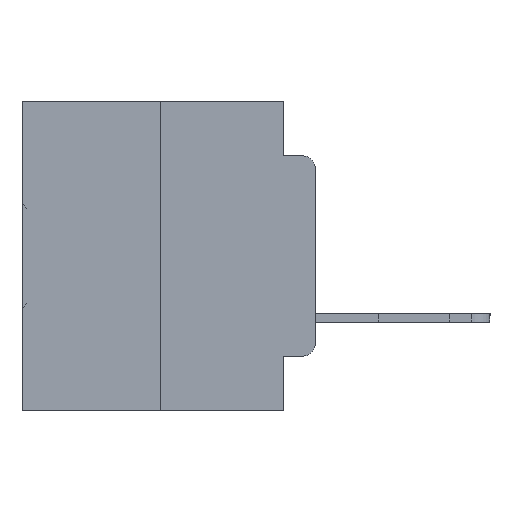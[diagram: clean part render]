
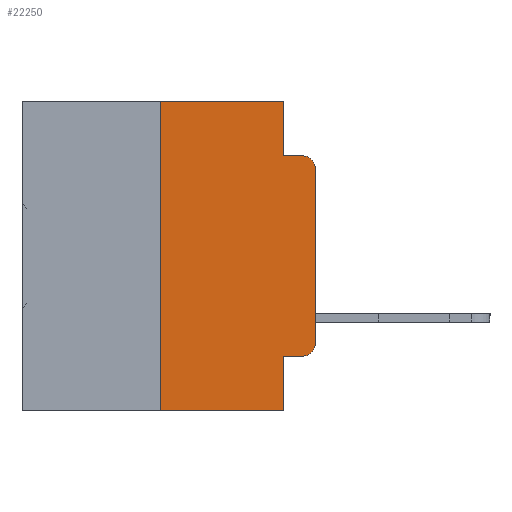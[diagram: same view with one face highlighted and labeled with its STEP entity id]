
A CAD part, left-side view. The second image highlights one B-rep face of the part: STEP entity #22250.
In plain terms, the highlighted planar face has unit normal (-1, 0, 0).
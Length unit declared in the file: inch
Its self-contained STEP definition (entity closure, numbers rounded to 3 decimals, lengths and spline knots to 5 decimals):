
#383 = CARTESIAN_POINT ( 'NONE',  ( 0., 0., -0.1085 ) ) ;
#525 = PLANE ( 'NONE',  #16255 ) ;
#553 = CARTESIAN_POINT ( 'NONE',  ( 0., 0.02, -0.3915 ) ) ;
#1141 = EDGE_CURVE ( 'NONE', #23824, #31234, #19177, .T. ) ;
#1585 = DIRECTION ( 'NONE',  ( 0., -1., 0. ) ) ;
#1615 = FACE_OUTER_BOUND ( 'NONE', #7427, .T. ) ;
#2001 = VECTOR ( 'NONE', #4054, 39.37008 ) ;
#2354 = ORIENTED_EDGE ( 'NONE', *, *, #4881, .T. ) ;
#2750 = VERTEX_POINT ( 'NONE', #25163 ) ;
#2858 = LINE ( 'NONE', #28061, #2001 ) ;
#3004 = EDGE_CURVE ( 'NONE', #31234, #20002, #31728, .T. ) ;
#3351 = DIRECTION ( 'NONE',  ( 0., 0., -1. ) ) ;
#3569 = DIRECTION ( 'NONE',  ( 0., 0., -1. ) ) ;
#4054 = DIRECTION ( 'NONE',  ( 0., 0., 1. ) ) ;
#4753 = VECTOR ( 'NONE', #26905, 39.37008 ) ;
#4881 = EDGE_CURVE ( 'NONE', #18666, #20002, #23552, .T. ) ;
#5510 = DIRECTION ( 'NONE',  ( -1., 0., 0. ) ) ;
#5546 = CARTESIAN_POINT ( 'NONE',  ( 0., 0.051, 0. ) ) ;
#5762 = CARTESIAN_POINT ( 'NONE',  ( 0., 0., 0. ) ) ;
#6622 = VECTOR ( 'NONE', #24027, 39.37008 ) ;
#6734 = EDGE_CURVE ( 'NONE', #2750, #18666, #7289, .T. ) ;
#7289 = LINE ( 'NONE', #5762, #8996 ) ;
#7427 = EDGE_LOOP ( 'NONE', ( #26678, #2354, #27138, #8411, #12592, #12186, #31841, #19689, #21334, #31044 ) ) ;
#8411 = ORIENTED_EDGE ( 'NONE', *, *, #1141, .F. ) ;
#8996 = VECTOR ( 'NONE', #24413, 39.37008 ) ;
#9454 = LINE ( 'NONE', #23056, #22681 ) ;
#9688 = VECTOR ( 'NONE', #33316, 39.37008 ) ;
#10018 = CIRCLE ( 'NONE', #17502, 0.02 ) ;
#11659 = CARTESIAN_POINT ( 'NONE',  ( 0., 0.473, 0. ) ) ;
#12150 = VECTOR ( 'NONE', #23650, 39.37008 ) ;
#12186 = ORIENTED_EDGE ( 'NONE', *, *, #30680, .F. ) ;
#12581 = EDGE_CURVE ( 'NONE', #21993, #22025, #9454, .T. ) ;
#12592 = ORIENTED_EDGE ( 'NONE', *, *, #18790, .F. ) ;
#13046 = CARTESIAN_POINT ( 'NONE',  ( 0., 0.051, 0. ) ) ;
#13049 = CARTESIAN_POINT ( 'NONE',  ( 0., 0.051, 0. ) ) ;
#14512 = CARTESIAN_POINT ( 'NONE',  ( 0., 0.473, 0. ) ) ;
#15523 = DIRECTION ( 'NONE',  ( 0., -1., 0. ) ) ;
#16255 = AXIS2_PLACEMENT_3D ( 'NONE', #11659, #19620, #3569 ) ;
#16707 = LINE ( 'NONE', #14512, #9688 ) ;
#16954 = AXIS2_PLACEMENT_3D ( 'NONE', #21490, #5510, #24166 ) ;
#17208 = CARTESIAN_POINT ( 'NONE',  ( 0., 0.02, -0.0885 ) ) ;
#17502 = AXIS2_PLACEMENT_3D ( 'NONE', #553, #19426, #3351 ) ;
#18666 = VERTEX_POINT ( 'NONE', #383 ) ;
#18790 = EDGE_CURVE ( 'NONE', #25694, #23824, #16707, .T. ) ;
#19177 = LINE ( 'NONE', #13046, #12150 ) ;
#19426 = DIRECTION ( 'NONE',  ( -1., 0., 0. ) ) ;
#19620 = DIRECTION ( 'NONE',  ( 1., 0., 0. ) ) ;
#19689 = ORIENTED_EDGE ( 'NONE', *, *, #28872, .F. ) ;
#19875 = EDGE_CURVE ( 'NONE', #29546, #2750, #10018, .T. ) ;
#19976 = CARTESIAN_POINT ( 'NONE',  ( 0., 0.051, -0.4115 ) ) ;
#20002 = VERTEX_POINT ( 'NONE', #17208 ) ;
#20763 = LINE ( 'NONE', #21333, #6622 ) ;
#21136 = CARTESIAN_POINT ( 'NONE',  ( 0., 0.25, -0.5 ) ) ;
#21247 = CARTESIAN_POINT ( 'NONE',  ( 0., 0.051, -0.5 ) ) ;
#21333 = CARTESIAN_POINT ( 'NONE',  ( 0., 0.051, -0.4115 ) ) ;
#21334 = ORIENTED_EDGE ( 'NONE', *, *, #27032, .T. ) ;
#21490 = CARTESIAN_POINT ( 'NONE',  ( 0., 0.02, -0.1085 ) ) ;
#21993 = VERTEX_POINT ( 'NONE', #21136 ) ;
#22025 = VERTEX_POINT ( 'NONE', #21247 ) ;
#22250 = ADVANCED_FACE ( 'NONE', ( #1615 ), #525, .F. ) ;
#22681 = VECTOR ( 'NONE', #1585, 39.37008 ) ;
#23056 = CARTESIAN_POINT ( 'NONE',  ( 0., 0.473, -0.5 ) ) ;
#23552 = CIRCLE ( 'NONE', #16954, 0.02 ) ;
#23650 = DIRECTION ( 'NONE',  ( 0., 0., -1. ) ) ;
#23824 = VERTEX_POINT ( 'NONE', #13049 ) ;
#24027 = DIRECTION ( 'NONE',  ( 0., -1., 0. ) ) ;
#24166 = DIRECTION ( 'NONE',  ( 0., 0., -1. ) ) ;
#24413 = DIRECTION ( 'NONE',  ( 0., 0., 1. ) ) ;
#24902 = VERTEX_POINT ( 'NONE', #19976 ) ;
#25163 = CARTESIAN_POINT ( 'NONE',  ( 0., 0., -0.3915 ) ) ;
#25694 = VERTEX_POINT ( 'NONE', #29205 ) ;
#26678 = ORIENTED_EDGE ( 'NONE', *, *, #6734, .T. ) ;
#26905 = DIRECTION ( 'NONE',  ( 0., 0., -1. ) ) ;
#26979 = CARTESIAN_POINT ( 'NONE',  ( 0., 0.02, -0.4115 ) ) ;
#27032 = EDGE_CURVE ( 'NONE', #24902, #29546, #20763, .T. ) ;
#27138 = ORIENTED_EDGE ( 'NONE', *, *, #3004, .F. ) ;
#27792 = CARTESIAN_POINT ( 'NONE',  ( 0., 0.051, -0.0885 ) ) ;
#28061 = CARTESIAN_POINT ( 'NONE',  ( 0., 0.25, 0. ) ) ;
#28872 = EDGE_CURVE ( 'NONE', #24902, #22025, #33236, .T. ) ;
#29205 = CARTESIAN_POINT ( 'NONE',  ( 0., 0.25, 0. ) ) ;
#29546 = VERTEX_POINT ( 'NONE', #26979 ) ;
#30680 = EDGE_CURVE ( 'NONE', #21993, #25694, #2858, .T. ) ;
#31044 = ORIENTED_EDGE ( 'NONE', *, *, #19875, .T. ) ;
#31234 = VERTEX_POINT ( 'NONE', #27792 ) ;
#31728 = LINE ( 'NONE', #34384, #32542 ) ;
#31841 = ORIENTED_EDGE ( 'NONE', *, *, #12581, .T. ) ;
#32542 = VECTOR ( 'NONE', #15523, 39.37008 ) ;
#33236 = LINE ( 'NONE', #5546, #4753 ) ;
#33316 = DIRECTION ( 'NONE',  ( 0., -1., 0. ) ) ;
#34384 = CARTESIAN_POINT ( 'NONE',  ( 0., 0.051, -0.0885 ) ) ;
